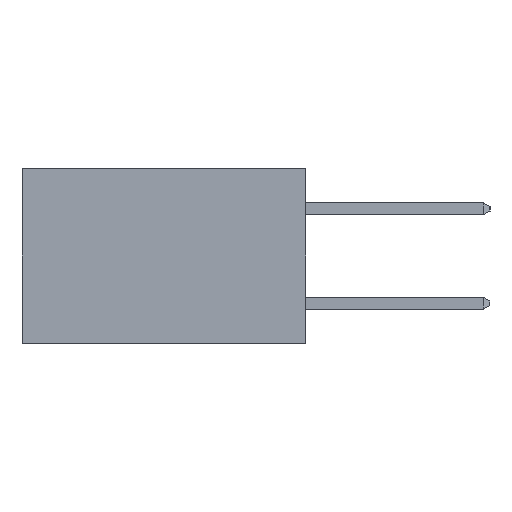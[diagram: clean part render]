
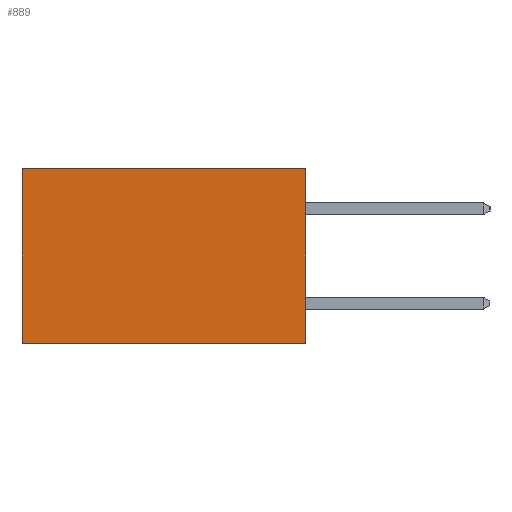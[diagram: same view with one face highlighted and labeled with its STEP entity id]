
A CAD part, left-side view. The second image highlights one B-rep face of the part: STEP entity #889.
In plain terms, the highlighted planar face has unit normal (-1, 0, 0).
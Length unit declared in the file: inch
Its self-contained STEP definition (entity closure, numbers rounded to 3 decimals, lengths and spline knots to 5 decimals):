
#889 = ADVANCED_FACE ( 'NONE', ( #2791 ), #4885, .F. ) ;
#2229 = DIRECTION ( 'NONE',  ( 1., 0., 0. ) ) ;
#2596 = DIRECTION ( 'NONE',  ( 0., 0., -1. ) ) ;
#2787 = DIRECTION ( 'NONE',  ( 0., 0., -1. ) ) ;
#2791 = FACE_OUTER_BOUND ( 'NONE', #23469, .T. ) ;
#3348 = ORIENTED_EDGE ( 'NONE', *, *, #26624, .F. ) ;
#3661 = CARTESIAN_POINT ( 'NONE',  ( 0.298, 0., 0. ) ) ;
#4520 = VECTOR ( 'NONE', #24817, 39.37008 ) ;
#4538 = VERTEX_POINT ( 'NONE', #26030 ) ;
#4885 = PLANE ( 'NONE',  #9247 ) ;
#5192 = LINE ( 'NONE', #22755, #4520 ) ;
#5311 = CARTESIAN_POINT ( 'NONE',  ( 0.298, 0., 0. ) ) ;
#5688 = DIRECTION ( 'NONE',  ( 0., 0., -1. ) ) ;
#5813 = VERTEX_POINT ( 'NONE', #26137 ) ;
#7248 = ORIENTED_EDGE ( 'NONE', *, *, #19601, .T. ) ;
#8352 = LINE ( 'NONE', #23681, #13341 ) ;
#8393 = DIRECTION ( 'NONE',  ( 0., 1., 0. ) ) ;
#9247 = AXIS2_PLACEMENT_3D ( 'NONE', #5311, #2229, #2596 ) ;
#9608 = VECTOR ( 'NONE', #5688, 39.37008 ) ;
#10492 = ORIENTED_EDGE ( 'NONE', *, *, #17901, .T. ) ;
#10921 = VERTEX_POINT ( 'NONE', #17499 ) ;
#13341 = VECTOR ( 'NONE', #2787, 39.37008 ) ;
#15791 = ORIENTED_EDGE ( 'NONE', *, *, #20649, .F. ) ;
#16815 = LINE ( 'NONE', #24968, #27089 ) ;
#17499 = CARTESIAN_POINT ( 'NONE',  ( 0.298, 0., -0.37 ) ) ;
#17901 = EDGE_CURVE ( 'NONE', #5813, #4538, #25524, .T. ) ;
#19601 = EDGE_CURVE ( 'NONE', #22009, #5813, #5192, .T. ) ;
#20355 = CARTESIAN_POINT ( 'NONE',  ( 0.298, 0.6, 0. ) ) ;
#20649 = EDGE_CURVE ( 'NONE', #22009, #10921, #8352, .T. ) ;
#22009 = VERTEX_POINT ( 'NONE', #3661 ) ;
#22755 = CARTESIAN_POINT ( 'NONE',  ( 0.298, 0., 0. ) ) ;
#23469 = EDGE_LOOP ( 'NONE', ( #10492, #3348, #15791, #7248 ) ) ;
#23681 = CARTESIAN_POINT ( 'NONE',  ( 0.298, 0., 0. ) ) ;
#24817 = DIRECTION ( 'NONE',  ( 0., 1., 0. ) ) ;
#24968 = CARTESIAN_POINT ( 'NONE',  ( 0.298, 0., -0.37 ) ) ;
#25524 = LINE ( 'NONE', #20355, #9608 ) ;
#26030 = CARTESIAN_POINT ( 'NONE',  ( 0.298, 0.6, -0.37 ) ) ;
#26137 = CARTESIAN_POINT ( 'NONE',  ( 0.298, 0.6, 0. ) ) ;
#26624 = EDGE_CURVE ( 'NONE', #10921, #4538, #16815, .T. ) ;
#27089 = VECTOR ( 'NONE', #8393, 39.37008 ) ;
